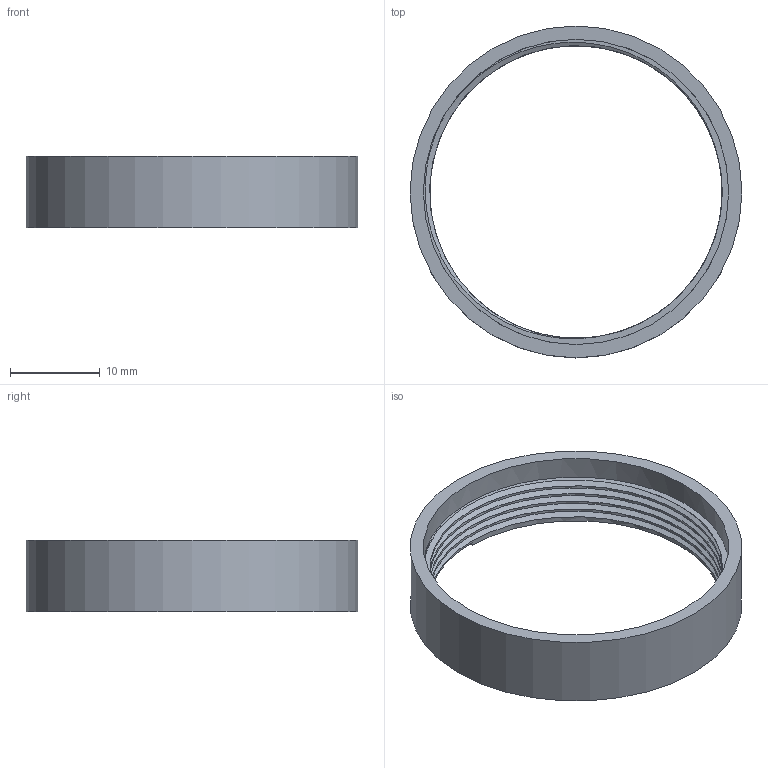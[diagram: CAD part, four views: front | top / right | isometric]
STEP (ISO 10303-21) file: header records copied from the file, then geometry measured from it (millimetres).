
FILE_DESCRIPTION (( 'STEP AP214' ), '1' );
FILE_NAME ('lockring.step', '2016-02-01T19:14:49', ( 'WarFairy' ), ( '' ), 'SwSTEP 2.0', 'SolidWorks 2015', '' );
FILE_SCHEMA (( 'AUTOMOTIVE_DESIGN' ));
Length unit declared in the file: inch
Products named in the file (1): lockring
Bounding box: 37.08 x 37.08 x 8 mm (x, y, z)
Volume: 1462.6 mm3; surface area: 2645.7 mm2
Topology: 1 solids, 1 shells, 9 faces, 17 edges, 11 vertices
Faces by surface type: plane 4, cylinder 3, bspline 2
Full cylindrical faces by diameter (mm): 34.112 x1, 37.084 x1
Entity records: 993 total; most frequent: CARTESIAN_POINT 789, DIRECTION 31, ORIENTED_EDGE 30, EDGE_CURVE 15, AXIS2_PLACEMENT_3D 14, EDGE_LOOP 14, FACE_OUTER_BOUND 11, VERTEX_POINT 11
